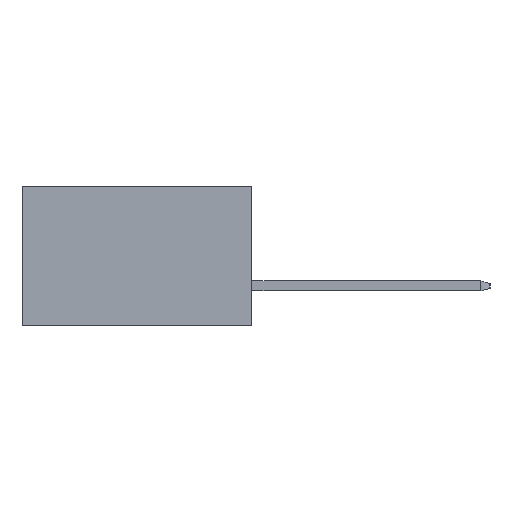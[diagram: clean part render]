
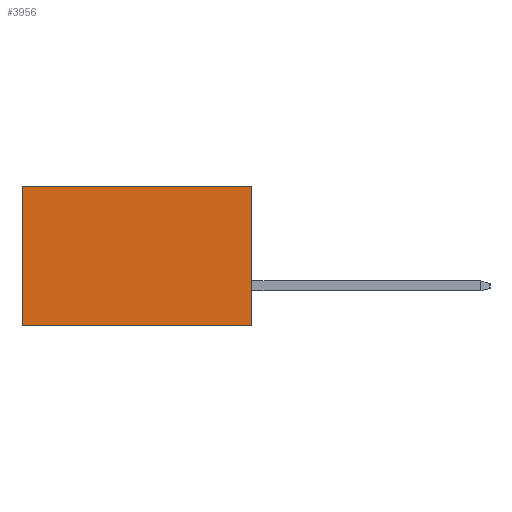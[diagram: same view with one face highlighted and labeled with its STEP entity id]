
A CAD part, left-side view. The second image highlights one B-rep face of the part: STEP entity #3956.
In plain terms, the highlighted planar face has unit normal (-1, 0, 0).
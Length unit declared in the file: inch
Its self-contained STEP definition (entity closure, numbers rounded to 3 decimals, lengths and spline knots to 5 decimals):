
#134 = DIRECTION ( 'NONE',  ( 0., 0., -1. ) ) ;
#235 = ORIENTED_EDGE ( 'NONE', *, *, #1607, .F. ) ;
#305 = VERTEX_POINT ( 'NONE', #5376 ) ;
#358 = ORIENTED_EDGE ( 'NONE', *, *, #7095, .T. ) ;
#378 = VECTOR ( 'NONE', #10159, 39.37008 ) ;
#642 = VERTEX_POINT ( 'NONE', #8966 ) ;
#1020 = CARTESIAN_POINT ( 'NONE',  ( 0.3205, 0., -0.437 ) ) ;
#1607 = EDGE_CURVE ( 'NONE', #9561, #1687, #9943, .T. ) ;
#1631 = ORIENTED_EDGE ( 'NONE', *, *, #11330, .T. ) ;
#1687 = VERTEX_POINT ( 'NONE', #5224 ) ;
#1905 = CARTESIAN_POINT ( 'NONE',  ( 0.3205, 0., 0. ) ) ;
#2204 = CARTESIAN_POINT ( 'NONE',  ( 0.3205, 0., 0. ) ) ;
#2589 = CARTESIAN_POINT ( 'NONE',  ( 0.3205, 0.72, -0.437 ) ) ;
#3956 = ADVANCED_FACE ( 'NONE', ( #10919 ), #5491, .F. ) ;
#3999 = DIRECTION ( 'NONE',  ( 0., 1., 0. ) ) ;
#4171 = LINE ( 'NONE', #2589, #4288 ) ;
#4288 = VECTOR ( 'NONE', #6190, 39.37008 ) ;
#4597 = DIRECTION ( 'NONE',  ( 1., 0., 0. ) ) ;
#4617 = EDGE_LOOP ( 'NONE', ( #1631, #8937, #235, #358 ) ) ;
#5224 = CARTESIAN_POINT ( 'NONE',  ( 0.3205, 0., -0.437 ) ) ;
#5376 = CARTESIAN_POINT ( 'NONE',  ( 0.3205, 0.72, 0. ) ) ;
#5491 = PLANE ( 'NONE',  #7820 ) ;
#5838 = LINE ( 'NONE', #6723, #10685 ) ;
#6190 = DIRECTION ( 'NONE',  ( 0., 0., -1. ) ) ;
#6723 = CARTESIAN_POINT ( 'NONE',  ( 0.3205, 0., -0.437 ) ) ;
#7095 = EDGE_CURVE ( 'NONE', #9561, #305, #10270, .T. ) ;
#7123 = DIRECTION ( 'NONE',  ( 0., 0., -1. ) ) ;
#7820 = AXIS2_PLACEMENT_3D ( 'NONE', #1020, #4597, #134 ) ;
#8559 = EDGE_CURVE ( 'NONE', #1687, #642, #5838, .T. ) ;
#8937 = ORIENTED_EDGE ( 'NONE', *, *, #8559, .F. ) ;
#8966 = CARTESIAN_POINT ( 'NONE',  ( 0.3205, 0.72, -0.437 ) ) ;
#9561 = VERTEX_POINT ( 'NONE', #1905 ) ;
#9884 = CARTESIAN_POINT ( 'NONE',  ( 0.3205, 0., -0.437 ) ) ;
#9943 = LINE ( 'NONE', #9884, #10370 ) ;
#10159 = DIRECTION ( 'NONE',  ( 0., 1., 0. ) ) ;
#10270 = LINE ( 'NONE', #2204, #378 ) ;
#10370 = VECTOR ( 'NONE', #7123, 39.37008 ) ;
#10685 = VECTOR ( 'NONE', #3999, 39.37008 ) ;
#10919 = FACE_OUTER_BOUND ( 'NONE', #4617, .T. ) ;
#11330 = EDGE_CURVE ( 'NONE', #305, #642, #4171, .T. ) ;
